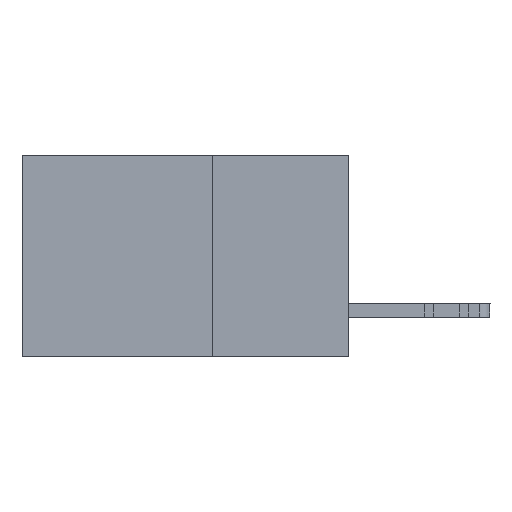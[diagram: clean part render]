
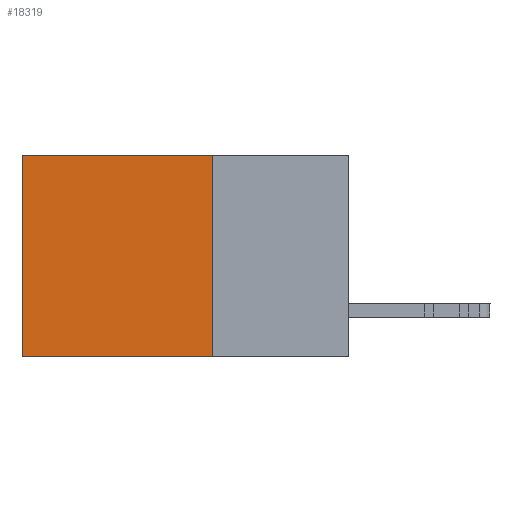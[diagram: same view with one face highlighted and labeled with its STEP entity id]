
A CAD part, left-side view. The second image highlights one B-rep face of the part: STEP entity #18319.
In plain terms, the highlighted planar face has unit normal (-1, 0, 0).
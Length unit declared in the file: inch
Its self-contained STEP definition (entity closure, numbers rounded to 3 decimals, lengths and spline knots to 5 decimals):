
#1625 = VECTOR ( 'NONE', #11988, 39.37008 ) ;
#3285 = EDGE_CURVE ( 'NONE', #15514, #4305, #16325, .T. ) ;
#3639 = ORIENTED_EDGE ( 'NONE', *, *, #14122, .T. ) ;
#4305 = VERTEX_POINT ( 'NONE', #13793 ) ;
#4341 = EDGE_LOOP ( 'NONE', ( #11656, #6243, #18595, #3639 ) ) ;
#4772 = CARTESIAN_POINT ( 'NONE',  ( 0.2615, 0.25, -0.37 ) ) ;
#6243 = ORIENTED_EDGE ( 'NONE', *, *, #3285, .F. ) ;
#7148 = VERTEX_POINT ( 'NONE', #17293 ) ;
#8993 = LINE ( 'NONE', #9670, #21004 ) ;
#9058 = EDGE_CURVE ( 'NONE', #15122, #4305, #10214, .T. ) ;
#9131 = DIRECTION ( 'NONE',  ( 0., 0., -1. ) ) ;
#9670 = CARTESIAN_POINT ( 'NONE',  ( 0.2615, 0.25, -0.37 ) ) ;
#10214 = LINE ( 'NONE', #16944, #19357 ) ;
#11190 = VECTOR ( 'NONE', #12710, 39.37008 ) ;
#11656 = ORIENTED_EDGE ( 'NONE', *, *, #9058, .T. ) ;
#11886 = CARTESIAN_POINT ( 'NONE',  ( 0.2615, 0.25, 0. ) ) ;
#11949 = AXIS2_PLACEMENT_3D ( 'NONE', #12726, #12678, #12654 ) ;
#11988 = DIRECTION ( 'NONE',  ( 0., 1., 0. ) ) ;
#12495 = CARTESIAN_POINT ( 'NONE',  ( 0.2615, 0.25, -0.37 ) ) ;
#12654 = DIRECTION ( 'NONE',  ( 0., 0., -1. ) ) ;
#12678 = DIRECTION ( 'NONE',  ( 1., 0., 0. ) ) ;
#12710 = DIRECTION ( 'NONE',  ( 0., 1., 0. ) ) ;
#12726 = CARTESIAN_POINT ( 'NONE',  ( 0.2615, 0.25, -0.37 ) ) ;
#12806 = PLANE ( 'NONE',  #11949 ) ;
#13515 = FACE_OUTER_BOUND ( 'NONE', #4341, .T. ) ;
#13793 = CARTESIAN_POINT ( 'NONE',  ( 0.2615, 0.6, -0.37 ) ) ;
#14122 = EDGE_CURVE ( 'NONE', #7148, #15122, #20049, .T. ) ;
#15122 = VERTEX_POINT ( 'NONE', #16814 ) ;
#15374 = EDGE_CURVE ( 'NONE', #7148, #15514, #8993, .T. ) ;
#15514 = VERTEX_POINT ( 'NONE', #4772 ) ;
#16325 = LINE ( 'NONE', #12495, #11190 ) ;
#16814 = CARTESIAN_POINT ( 'NONE',  ( 0.2615, 0.6, 0. ) ) ;
#16916 = DIRECTION ( 'NONE',  ( 0., 0., -1. ) ) ;
#16944 = CARTESIAN_POINT ( 'NONE',  ( 0.2615, 0.6, -0.37 ) ) ;
#17293 = CARTESIAN_POINT ( 'NONE',  ( 0.2615, 0.25, 0. ) ) ;
#18319 = ADVANCED_FACE ( 'NONE', ( #13515 ), #12806, .F. ) ;
#18595 = ORIENTED_EDGE ( 'NONE', *, *, #15374, .F. ) ;
#19357 = VECTOR ( 'NONE', #16916, 39.37008 ) ;
#20049 = LINE ( 'NONE', #11886, #1625 ) ;
#21004 = VECTOR ( 'NONE', #9131, 39.37008 ) ;
